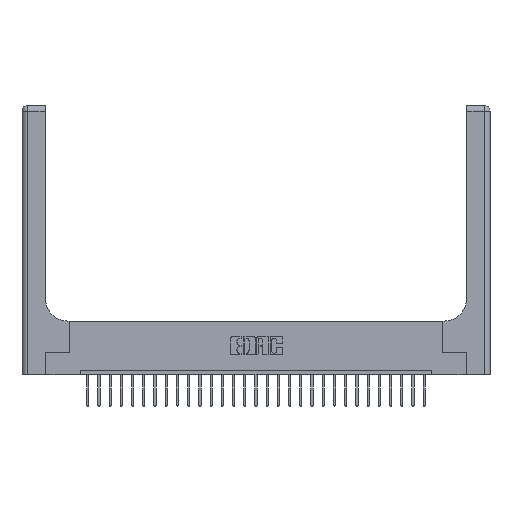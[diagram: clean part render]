
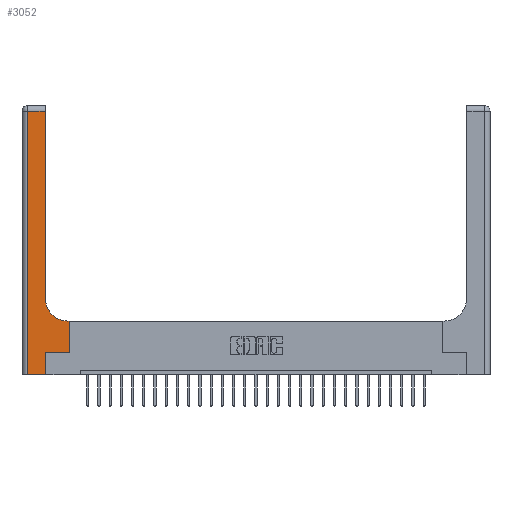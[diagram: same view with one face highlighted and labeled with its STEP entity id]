
A CAD part, top view. The second image highlights one B-rep face of the part: STEP entity #3052.
In plain terms, the highlighted planar face has unit normal (0, 0, 1).
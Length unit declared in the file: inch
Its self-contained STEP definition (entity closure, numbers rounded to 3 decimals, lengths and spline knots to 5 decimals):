
#1065 = LINE ( 'NONE', #1513, #16830 ) ;
#1513 = CARTESIAN_POINT ( 'NONE',  ( 0., 0., 0.37 ) ) ;
#1770 = DIRECTION ( 'NONE',  ( 0., 1., 0. ) ) ;
#2393 = PLANE ( 'NONE',  #24719 ) ;
#2831 = VERTEX_POINT ( 'NONE', #10802 ) ;
#3052 = ADVANCED_FACE ( 'NONE', ( #16104 ), #2393, .F. ) ;
#3087 = VERTEX_POINT ( 'NONE', #11713 ) ;
#4385 = EDGE_CURVE ( 'NONE', #23750, #16863, #25636, .T. ) ;
#4640 = VERTEX_POINT ( 'NONE', #9422 ) ;
#5488 = CARTESIAN_POINT ( 'NONE',  ( 0.51, 0.85, 0.37 ) ) ;
#6526 = ORIENTED_EDGE ( 'NONE', *, *, #24464, .T. ) ;
#6814 = ORIENTED_EDGE ( 'NONE', *, *, #14760, .T. ) ;
#6850 = DIRECTION ( 'NONE',  ( 0., 0., -1. ) ) ;
#7166 = ORIENTED_EDGE ( 'NONE', *, *, #22628, .T. ) ;
#7577 = EDGE_CURVE ( 'NONE', #14550, #2831, #24071, .T. ) ;
#8019 = CARTESIAN_POINT ( 'NONE',  ( 0.26, 0.6, 0.37 ) ) ;
#8034 = CARTESIAN_POINT ( 'NONE',  ( 0.06, 3., 0.37 ) ) ;
#8150 = LINE ( 'NONE', #11038, #20734 ) ;
#8584 = ORIENTED_EDGE ( 'NONE', *, *, #7577, .T. ) ;
#8700 = VECTOR ( 'NONE', #1770, 39.37008 ) ;
#8703 = CARTESIAN_POINT ( 'NONE',  ( 0.265, 0., 0.37 ) ) ;
#9140 = DIRECTION ( 'NONE',  ( 1., 0., 0. ) ) ;
#9170 = ORIENTED_EDGE ( 'NONE', *, *, #22098, .T. ) ;
#9263 = VERTEX_POINT ( 'NONE', #15475 ) ;
#9422 = CARTESIAN_POINT ( 'NONE',  ( 0.51, 0.6, 0.37 ) ) ;
#9473 = DIRECTION ( 'NONE',  ( 1., 0., 0. ) ) ;
#9681 = VECTOR ( 'NONE', #14402, 39.37008 ) ;
#9746 = CARTESIAN_POINT ( 'NONE',  ( 0., 2.94, 0.37 ) ) ;
#9781 = VECTOR ( 'NONE', #10133, 39.37008 ) ;
#9872 = CARTESIAN_POINT ( 'NONE',  ( 0.06, 2.94, 0.37 ) ) ;
#9929 = EDGE_CURVE ( 'NONE', #25343, #23750, #1065, .T. ) ;
#10133 = DIRECTION ( 'NONE',  ( -1., 0., 0. ) ) ;
#10448 = EDGE_LOOP ( 'NONE', ( #8584, #22623, #12869, #24279, #11657, #6526, #6814, #7166, #9170 ) ) ;
#10452 = AXIS2_PLACEMENT_3D ( 'NONE', #5488, #25277, #9473 ) ;
#10802 = CARTESIAN_POINT ( 'NONE',  ( 0.26, 2.94, 0.37 ) ) ;
#10850 = DIRECTION ( 'NONE',  ( 1., 0., 0. ) ) ;
#10853 = CARTESIAN_POINT ( 'NONE',  ( 0., 3., 0.37 ) ) ;
#11038 = CARTESIAN_POINT ( 'NONE',  ( 0.265, 0.25, 0.37 ) ) ;
#11657 = ORIENTED_EDGE ( 'NONE', *, *, #4385, .T. ) ;
#11713 = CARTESIAN_POINT ( 'NONE',  ( 0.528, 0.25, 0.37 ) ) ;
#11841 = CARTESIAN_POINT ( 'NONE',  ( 0.26, 3., 0.37 ) ) ;
#12850 = LINE ( 'NONE', #8034, #13783 ) ;
#12869 = ORIENTED_EDGE ( 'NONE', *, *, #20242, .T. ) ;
#13385 = CIRCLE ( 'NONE', #10452, 0.25 ) ;
#13783 = VECTOR ( 'NONE', #17486, 39.37008 ) ;
#14402 = DIRECTION ( 'NONE',  ( 0., 1., 0. ) ) ;
#14550 = VERTEX_POINT ( 'NONE', #15064 ) ;
#14760 = EDGE_CURVE ( 'NONE', #3087, #9263, #21038, .T. ) ;
#15064 = CARTESIAN_POINT ( 'NONE',  ( 0.26, 0.85, 0.37 ) ) ;
#15475 = CARTESIAN_POINT ( 'NONE',  ( 0.528, 0.6, 0.37 ) ) ;
#16104 = FACE_OUTER_BOUND ( 'NONE', #10448, .T. ) ;
#16485 = LINE ( 'NONE', #8019, #9781 ) ;
#16830 = VECTOR ( 'NONE', #9140, 39.37008 ) ;
#16863 = VERTEX_POINT ( 'NONE', #18863 ) ;
#17486 = DIRECTION ( 'NONE',  ( 0., -1., 0. ) ) ;
#17905 = EDGE_CURVE ( 'NONE', #2831, #21985, #18664, .T. ) ;
#18098 = DIRECTION ( 'NONE',  ( -1., 0., 0. ) ) ;
#18664 = LINE ( 'NONE', #9746, #20447 ) ;
#18863 = CARTESIAN_POINT ( 'NONE',  ( 0.265, 0.25, 0.37 ) ) ;
#18880 = DIRECTION ( 'NONE',  ( 0., 1., 0. ) ) ;
#20242 = EDGE_CURVE ( 'NONE', #21985, #25343, #12850, .T. ) ;
#20260 = CARTESIAN_POINT ( 'NONE',  ( 0.265, 0., 0.37 ) ) ;
#20347 = VECTOR ( 'NONE', #18880, 39.37008 ) ;
#20447 = VECTOR ( 'NONE', #18098, 39.37008 ) ;
#20734 = VECTOR ( 'NONE', #10850, 39.37008 ) ;
#21038 = LINE ( 'NONE', #23966, #9681 ) ;
#21985 = VERTEX_POINT ( 'NONE', #9872 ) ;
#22098 = EDGE_CURVE ( 'NONE', #4640, #14550, #13385, .T. ) ;
#22623 = ORIENTED_EDGE ( 'NONE', *, *, #17905, .T. ) ;
#22628 = EDGE_CURVE ( 'NONE', #9263, #4640, #16485, .T. ) ;
#22980 = DIRECTION ( 'NONE',  ( -1., 0., 0. ) ) ;
#23750 = VERTEX_POINT ( 'NONE', #20260 ) ;
#23777 = CARTESIAN_POINT ( 'NONE',  ( 0.06, 0., 0.37 ) ) ;
#23966 = CARTESIAN_POINT ( 'NONE',  ( 0.528, 0.25, 0.37 ) ) ;
#24071 = LINE ( 'NONE', #11841, #8700 ) ;
#24279 = ORIENTED_EDGE ( 'NONE', *, *, #9929, .T. ) ;
#24464 = EDGE_CURVE ( 'NONE', #16863, #3087, #8150, .T. ) ;
#24719 = AXIS2_PLACEMENT_3D ( 'NONE', #10853, #6850, #22980 ) ;
#25277 = DIRECTION ( 'NONE',  ( 0., 0., -1. ) ) ;
#25343 = VERTEX_POINT ( 'NONE', #23777 ) ;
#25636 = LINE ( 'NONE', #8703, #20347 ) ;
